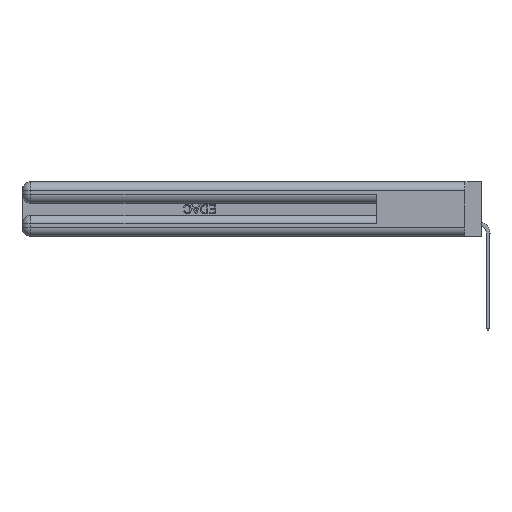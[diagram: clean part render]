
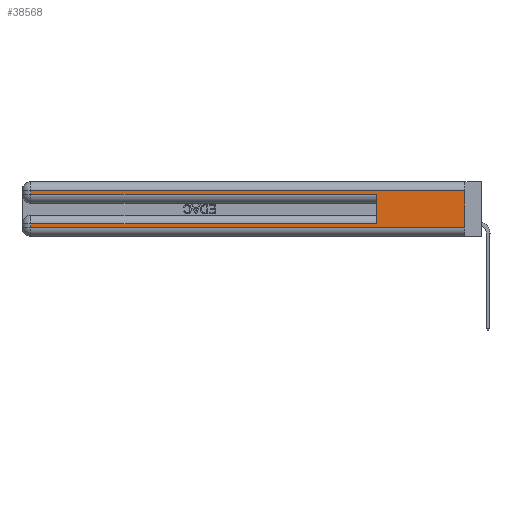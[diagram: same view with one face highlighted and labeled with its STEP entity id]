
A CAD part, left-side view. The second image highlights one B-rep face of the part: STEP entity #38568.
In plain terms, the highlighted planar face has unit normal (-1, 0, 0).
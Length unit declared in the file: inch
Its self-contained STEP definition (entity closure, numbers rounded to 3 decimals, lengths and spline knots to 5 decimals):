
#863 = EDGE_CURVE ( 'NONE', #19423, #11801, #33493, .T. ) ;
#866 = CARTESIAN_POINT ( 'NONE',  ( 0., 0., 0.06 ) ) ;
#1262 = CARTESIAN_POINT ( 'NONE',  ( 0., 0., 0.085 ) ) ;
#1880 = VECTOR ( 'NONE', #28083, 39.37008 ) ;
#1976 = VECTOR ( 'NONE', #16944, 39.37008 ) ;
#2452 = ORIENTED_EDGE ( 'NONE', *, *, #9885, .T. ) ;
#3017 = CARTESIAN_POINT ( 'NONE',  ( 0., 2.94, 0.37 ) ) ;
#3138 = ORIENTED_EDGE ( 'NONE', *, *, #18750, .T. ) ;
#3426 = EDGE_CURVE ( 'NONE', #35539, #11801, #31632, .T. ) ;
#4656 = CARTESIAN_POINT ( 'NONE',  ( 0., 0., 0.285 ) ) ;
#5761 = ORIENTED_EDGE ( 'NONE', *, *, #29609, .T. ) ;
#6413 = LINE ( 'NONE', #10245, #31258 ) ;
#6487 = CARTESIAN_POINT ( 'NONE',  ( 0., 0., 0.37 ) ) ;
#7658 = EDGE_LOOP ( 'NONE', ( #16005, #10999, #3138, #31660, #30527, #2452, #5761, #18704 ) ) ;
#9885 = EDGE_CURVE ( 'NONE', #19423, #13595, #34055, .T. ) ;
#9941 = DIRECTION ( 'NONE',  ( 0., 1., 0. ) ) ;
#10245 = CARTESIAN_POINT ( 'NONE',  ( 0., 0., 0.31 ) ) ;
#10760 = CARTESIAN_POINT ( 'NONE',  ( 0., 0., 0.37 ) ) ;
#10999 = ORIENTED_EDGE ( 'NONE', *, *, #30132, .T. ) ;
#11470 = AXIS2_PLACEMENT_3D ( 'NONE', #10760, #35491, #38595 ) ;
#11801 = VERTEX_POINT ( 'NONE', #16402 ) ;
#11862 = DIRECTION ( 'NONE',  ( 0., 0., -1. ) ) ;
#12443 = LINE ( 'NONE', #23599, #1976 ) ;
#12999 = DIRECTION ( 'NONE',  ( 0., 1., 0. ) ) ;
#13595 = VERTEX_POINT ( 'NONE', #16384 ) ;
#14391 = VECTOR ( 'NONE', #43690, 39.37008 ) ;
#14757 = CARTESIAN_POINT ( 'NONE',  ( 0., 0.6, 0.145 ) ) ;
#15668 = CARTESIAN_POINT ( 'NONE',  ( 0., 2.94, 0.31 ) ) ;
#16005 = ORIENTED_EDGE ( 'NONE', *, *, #40231, .F. ) ;
#16180 = VERTEX_POINT ( 'NONE', #866 ) ;
#16384 = CARTESIAN_POINT ( 'NONE',  ( 0., 2.94, 0.085 ) ) ;
#16402 = CARTESIAN_POINT ( 'NONE',  ( 0., 0.6, 0.285 ) ) ;
#16944 = DIRECTION ( 'NONE',  ( 0., -1., 0. ) ) ;
#18559 = FACE_OUTER_BOUND ( 'NONE', #7658, .T. ) ;
#18704 = ORIENTED_EDGE ( 'NONE', *, *, #25010, .T. ) ;
#18750 = EDGE_CURVE ( 'NONE', #24517, #35539, #35186, .T. ) ;
#19423 = VERTEX_POINT ( 'NONE', #36300 ) ;
#22972 = VECTOR ( 'NONE', #11862, 39.37008 ) ;
#23599 = CARTESIAN_POINT ( 'NONE',  ( 0., 0., 0.06 ) ) ;
#24445 = DIRECTION ( 'NONE',  ( 0., 0., -1. ) ) ;
#24517 = VERTEX_POINT ( 'NONE', #15668 ) ;
#24609 = VECTOR ( 'NONE', #12999, 39.37008 ) ;
#25010 = EDGE_CURVE ( 'NONE', #41584, #16180, #12443, .T. ) ;
#26341 = VECTOR ( 'NONE', #24445, 39.37008 ) ;
#28083 = DIRECTION ( 'NONE',  ( 0., 0., -1. ) ) ;
#29609 = EDGE_CURVE ( 'NONE', #13595, #41584, #38983, .T. ) ;
#30132 = EDGE_CURVE ( 'NONE', #40426, #24517, #6413, .T. ) ;
#30527 = ORIENTED_EDGE ( 'NONE', *, *, #863, .F. ) ;
#30733 = CARTESIAN_POINT ( 'NONE',  ( 0., 2.94, 0.06 ) ) ;
#31258 = VECTOR ( 'NONE', #9941, 39.37008 ) ;
#31632 = LINE ( 'NONE', #4656, #14391 ) ;
#31660 = ORIENTED_EDGE ( 'NONE', *, *, #3426, .T. ) ;
#32356 = VECTOR ( 'NONE', #36905, 39.37008 ) ;
#33493 = LINE ( 'NONE', #14757, #32356 ) ;
#34055 = LINE ( 'NONE', #1262, #24609 ) ;
#35186 = LINE ( 'NONE', #3017, #26341 ) ;
#35491 = DIRECTION ( 'NONE',  ( 1., 0., 0. ) ) ;
#35539 = VERTEX_POINT ( 'NONE', #42110 ) ;
#36300 = CARTESIAN_POINT ( 'NONE',  ( 0., 0.6, 0.085 ) ) ;
#36405 = CARTESIAN_POINT ( 'NONE',  ( 0., 2.94, 0.37 ) ) ;
#36905 = DIRECTION ( 'NONE',  ( 0., 0., 1. ) ) ;
#37780 = CARTESIAN_POINT ( 'NONE',  ( 0., 0., 0.31 ) ) ;
#38568 = ADVANCED_FACE ( 'NONE', ( #18559 ), #38725, .F. ) ;
#38595 = DIRECTION ( 'NONE',  ( 0., 0., -1. ) ) ;
#38725 = PLANE ( 'NONE',  #11470 ) ;
#38983 = LINE ( 'NONE', #36405, #22972 ) ;
#40231 = EDGE_CURVE ( 'NONE', #40426, #16180, #41644, .T. ) ;
#40426 = VERTEX_POINT ( 'NONE', #37780 ) ;
#41584 = VERTEX_POINT ( 'NONE', #30733 ) ;
#41644 = LINE ( 'NONE', #6487, #1880 ) ;
#42110 = CARTESIAN_POINT ( 'NONE',  ( 0., 2.94, 0.285 ) ) ;
#43690 = DIRECTION ( 'NONE',  ( 0., -1., 0. ) ) ;
